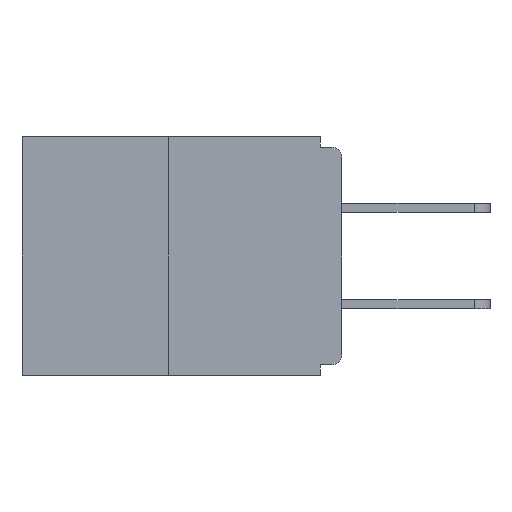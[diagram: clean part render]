
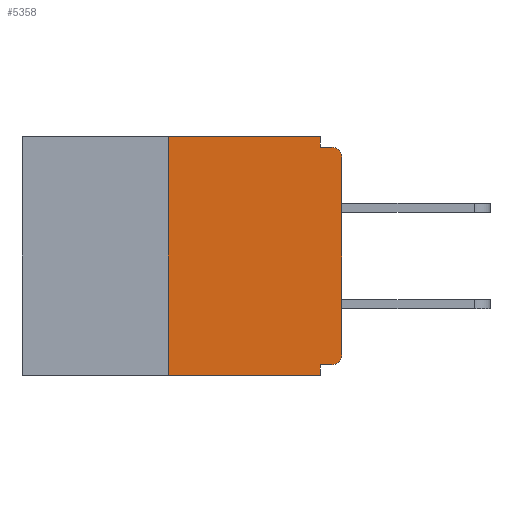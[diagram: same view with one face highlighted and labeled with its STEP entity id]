
A CAD part, left-side view. The second image highlights one B-rep face of the part: STEP entity #5358.
In plain terms, the highlighted planar face has unit normal (-1, 0, 0).
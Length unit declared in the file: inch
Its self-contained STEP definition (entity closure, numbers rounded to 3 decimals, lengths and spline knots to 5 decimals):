
#258 = CARTESIAN_POINT ( 'NONE',  ( 0., 0.015, -0.313 ) ) ;
#773 = CARTESIAN_POINT ( 'NONE',  ( 0., 0.015, -0.03 ) ) ;
#1032 = CARTESIAN_POINT ( 'NONE',  ( 0., 0.25, 0. ) ) ;
#1741 = CIRCLE ( 'NONE', #4475, 0.015 ) ;
#1855 = ORIENTED_EDGE ( 'NONE', *, *, #21075, .T. ) ;
#1964 = VERTEX_POINT ( 'NONE', #4230 ) ;
#2282 = EDGE_CURVE ( 'NONE', #5649, #17291, #7638, .T. ) ;
#2810 = DIRECTION ( 'NONE',  ( 0., 0., -1. ) ) ;
#3019 = EDGE_CURVE ( 'NONE', #5649, #5632, #15745, .T. ) ;
#3446 = LINE ( 'NONE', #15763, #21740 ) ;
#4028 = ORIENTED_EDGE ( 'NONE', *, *, #3019, .T. ) ;
#4230 = CARTESIAN_POINT ( 'NONE',  ( 0., 0.25, -0.343 ) ) ;
#4447 = EDGE_CURVE ( 'NONE', #27520, #24927, #3446, .T. ) ;
#4457 = VECTOR ( 'NONE', #14565, 39.37008 ) ;
#4475 = AXIS2_PLACEMENT_3D ( 'NONE', #773, #13492, #2810 ) ;
#5358 = ADVANCED_FACE ( 'NONE', ( #20324 ), #23048, .F. ) ;
#5466 = LINE ( 'NONE', #10211, #4457 ) ;
#5632 = VERTEX_POINT ( 'NONE', #24590 ) ;
#5649 = VERTEX_POINT ( 'NONE', #11958 ) ;
#5877 = VERTEX_POINT ( 'NONE', #26552 ) ;
#6061 = CARTESIAN_POINT ( 'NONE',  ( 0., 0.015, -0.015 ) ) ;
#6991 = DIRECTION ( 'NONE',  ( 0., -1., 0. ) ) ;
#7638 = LINE ( 'NONE', #8030, #15434 ) ;
#7685 = EDGE_CURVE ( 'NONE', #20187, #27520, #12648, .T. ) ;
#8030 = CARTESIAN_POINT ( 'NONE',  ( 0., 0., -0.328 ) ) ;
#8081 = DIRECTION ( 'NONE',  ( 0., 0., -1. ) ) ;
#8493 = VECTOR ( 'NONE', #21174, 39.37008 ) ;
#8697 = LINE ( 'NONE', #19182, #28055 ) ;
#8937 = AXIS2_PLACEMENT_3D ( 'NONE', #27424, #18880, #8081 ) ;
#9141 = LINE ( 'NONE', #14542, #8493 ) ;
#9196 = EDGE_CURVE ( 'NONE', #5632, #9414, #9141, .T. ) ;
#9414 = VERTEX_POINT ( 'NONE', #19347 ) ;
#9563 = CARTESIAN_POINT ( 'NONE',  ( 0., 0.031, -0.328 ) ) ;
#10211 = CARTESIAN_POINT ( 'NONE',  ( 0., 0.031, -0.343 ) ) ;
#11221 = DIRECTION ( 'NONE',  ( 0., 0., -1. ) ) ;
#11296 = VECTOR ( 'NONE', #13720, 39.37008 ) ;
#11958 = CARTESIAN_POINT ( 'NONE',  ( 0., 0.015, -0.328 ) ) ;
#12648 = LINE ( 'NONE', #24519, #11296 ) ;
#13492 = DIRECTION ( 'NONE',  ( -1., 0., 0. ) ) ;
#13720 = DIRECTION ( 'NONE',  ( 0., 0., -1. ) ) ;
#14032 = AXIS2_PLACEMENT_3D ( 'NONE', #258, #17088, #11221 ) ;
#14382 = LINE ( 'NONE', #15733, #19473 ) ;
#14542 = CARTESIAN_POINT ( 'NONE',  ( 0., 0., 0. ) ) ;
#14565 = DIRECTION ( 'NONE',  ( 0., 0., -1. ) ) ;
#15200 = DIRECTION ( 'NONE',  ( 0., -1., 0. ) ) ;
#15434 = VECTOR ( 'NONE', #21096, 39.37008 ) ;
#15733 = CARTESIAN_POINT ( 'NONE',  ( 0., 0.46, 0. ) ) ;
#15745 = CIRCLE ( 'NONE', #14032, 0.015 ) ;
#15763 = CARTESIAN_POINT ( 'NONE',  ( 0., 0., -0.015 ) ) ;
#15872 = CARTESIAN_POINT ( 'NONE',  ( 0., 0.031, 0. ) ) ;
#15927 = CARTESIAN_POINT ( 'NONE',  ( 0., 0.031, -0.015 ) ) ;
#15960 = DIRECTION ( 'NONE',  ( 0., 0., 1. ) ) ;
#16041 = DIRECTION ( 'NONE',  ( 0., -1., 0. ) ) ;
#17002 = VECTOR ( 'NONE', #15960, 39.37008 ) ;
#17069 = ORIENTED_EDGE ( 'NONE', *, *, #4447, .F. ) ;
#17088 = DIRECTION ( 'NONE',  ( -1., 0., 0. ) ) ;
#17291 = VERTEX_POINT ( 'NONE', #9563 ) ;
#18297 = EDGE_LOOP ( 'NONE', ( #27267, #26609, #1855, #25134, #21194, #4028, #26937, #27598, #17069, #22931 ) ) ;
#18803 = EDGE_CURVE ( 'NONE', #9414, #24927, #1741, .T. ) ;
#18880 = DIRECTION ( 'NONE',  ( 1., 0., 0. ) ) ;
#19182 = CARTESIAN_POINT ( 'NONE',  ( 0., 0.46, -0.343 ) ) ;
#19347 = CARTESIAN_POINT ( 'NONE',  ( 0., 0., -0.03 ) ) ;
#19473 = VECTOR ( 'NONE', #6991, 39.37008 ) ;
#20187 = VERTEX_POINT ( 'NONE', #15872 ) ;
#20324 = FACE_OUTER_BOUND ( 'NONE', #18297, .T. ) ;
#21075 = EDGE_CURVE ( 'NONE', #1964, #5877, #8697, .T. ) ;
#21096 = DIRECTION ( 'NONE',  ( 0., 1., 0. ) ) ;
#21174 = DIRECTION ( 'NONE',  ( 0., 0., 1. ) ) ;
#21194 = ORIENTED_EDGE ( 'NONE', *, *, #2282, .F. ) ;
#21740 = VECTOR ( 'NONE', #16041, 39.37008 ) ;
#22564 = EDGE_CURVE ( 'NONE', #27783, #20187, #14382, .T. ) ;
#22931 = ORIENTED_EDGE ( 'NONE', *, *, #7685, .F. ) ;
#23048 = PLANE ( 'NONE',  #8937 ) ;
#23184 = CARTESIAN_POINT ( 'NONE',  ( 0., 0.25, 0. ) ) ;
#23433 = LINE ( 'NONE', #1032, #17002 ) ;
#24014 = EDGE_CURVE ( 'NONE', #1964, #27783, #23433, .T. ) ;
#24519 = CARTESIAN_POINT ( 'NONE',  ( 0., 0.031, 0. ) ) ;
#24590 = CARTESIAN_POINT ( 'NONE',  ( 0., 0., -0.313 ) ) ;
#24927 = VERTEX_POINT ( 'NONE', #6061 ) ;
#25134 = ORIENTED_EDGE ( 'NONE', *, *, #25273, .F. ) ;
#25273 = EDGE_CURVE ( 'NONE', #17291, #5877, #5466, .T. ) ;
#26552 = CARTESIAN_POINT ( 'NONE',  ( 0., 0.031, -0.343 ) ) ;
#26609 = ORIENTED_EDGE ( 'NONE', *, *, #24014, .F. ) ;
#26937 = ORIENTED_EDGE ( 'NONE', *, *, #9196, .T. ) ;
#27267 = ORIENTED_EDGE ( 'NONE', *, *, #22564, .F. ) ;
#27424 = CARTESIAN_POINT ( 'NONE',  ( 0., 0.46, 0. ) ) ;
#27520 = VERTEX_POINT ( 'NONE', #15927 ) ;
#27598 = ORIENTED_EDGE ( 'NONE', *, *, #18803, .T. ) ;
#27783 = VERTEX_POINT ( 'NONE', #23184 ) ;
#28055 = VECTOR ( 'NONE', #15200, 39.37008 ) ;
